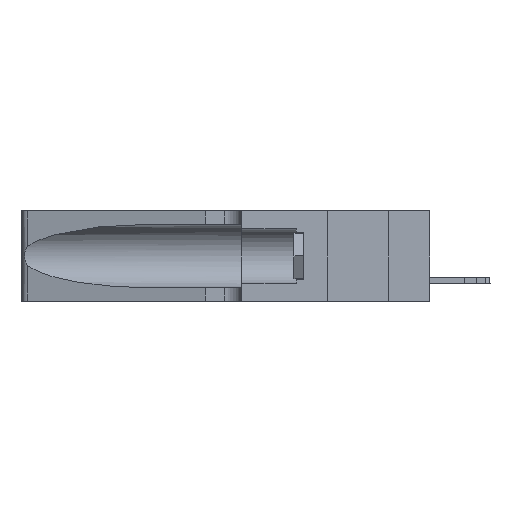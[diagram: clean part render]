
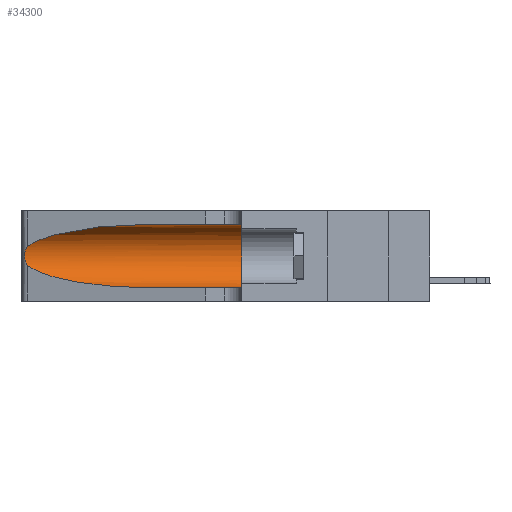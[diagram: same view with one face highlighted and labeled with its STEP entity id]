
A CAD part, left-side view. The second image highlights one B-rep face of the part: STEP entity #34300.
In plain terms, the highlighted cylindrical face has radius 3.308 mm (diameter 6.617 mm), a partial arc.
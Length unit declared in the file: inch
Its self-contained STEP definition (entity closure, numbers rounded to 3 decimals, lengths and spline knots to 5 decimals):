
#672 =( BOUNDED_CURVE ( )  B_SPLINE_CURVE ( 3, ( #29428, #14460, #37527, #17383 ),
 .UNSPECIFIED., .F., .F. ) 
 B_SPLINE_CURVE_WITH_KNOTS ( ( 4, 4 ),
 ( 1.5708, 2.84003 ),
 .UNSPECIFIED. ) 
 CURVE ( )  GEOMETRIC_REPRESENTATION_ITEM ( )  RATIONAL_B_SPLINE_CURVE ( ( 1., 0.87, 0.87, 1. ) ) 
 REPRESENTATION_ITEM ( '' )  );
#2337 = CARTESIAN_POINT ( 'NONE',  ( 0.1305, 1.61858, 0.31525 ) ) ;
#2649 = VERTEX_POINT ( 'NONE', #10686 ) ;
#4021 = CARTESIAN_POINT ( 'NONE',  ( 0.1305, 0.72297, 0.05475 ) ) ;
#5662 = VERTEX_POINT ( 'NONE', #19962 ) ;
#5851 = B_SPLINE_CURVE_WITH_KNOTS ( 'NONE', 3,
 ( #28450, #34926, #15930, #18313, #19242, #28976, #17989, #9977, #15608, #33112, #9560, #18122, #21887, #27722 ),
 .UNSPECIFIED., .F., .F.,
 ( 4, 2, 2, 2, 2, 2, 4 ),
 ( 0., 0.00027, 0.00053, 0.00107, 0.0016, 0.00187, 0.00214 ),
 .UNSPECIFIED. ) ;
#6387 = CARTESIAN_POINT ( 'NONE',  ( 0.1305, 1.61858, 0.185 ) ) ;
#6598 = CIRCLE ( 'NONE', #23271, 0.13025 ) ;
#6604 = ORIENTED_EDGE ( 'NONE', *, *, #36650, .T. ) ;
#7094 = VERTEX_POINT ( 'NONE', #14188 ) ;
#9121 = AXIS2_PLACEMENT_3D ( 'NONE', #6387, #23999, #16027 ) ;
#9560 = CARTESIAN_POINT ( 'NONE',  ( 0.25789, 1.23486, 0.15765 ) ) ;
#9602 = DIRECTION ( 'NONE',  ( 0., 1., 0. ) ) ;
#9977 = CARTESIAN_POINT ( 'NONE',  ( 0.26075, 1.23896, 0.178 ) ) ;
#10686 = CARTESIAN_POINT ( 'NONE',  ( 0.1305, 0.35, 0.05475 ) ) ;
#10847 = EDGE_CURVE ( 'NONE', #5662, #19562, #32777, .T. ) ;
#10902 = DIRECTION ( 'NONE',  ( 0., -1., 0. ) ) ;
#11139 = CARTESIAN_POINT ( 'NONE',  ( 0.1305, 1.61858, 0.05475 ) ) ;
#12680 = CARTESIAN_POINT ( 'NONE',  ( 0.25487, 1.22718, 0.22369 ) ) ;
#14188 = CARTESIAN_POINT ( 'NONE',  ( 0.1305, 0.72297, 0.31525 ) ) ;
#14238 = ORIENTED_EDGE ( 'NONE', *, *, #22538, .T. ) ;
#14460 = CARTESIAN_POINT ( 'NONE',  ( 0.18966, 0.96281, 0.31525 ) ) ;
#14892 = ORIENTED_EDGE ( 'NONE', *, *, #37406, .F. ) ;
#15608 = CARTESIAN_POINT ( 'NONE',  ( 0.26017, 1.23833, 0.17102 ) ) ;
#15930 = CARTESIAN_POINT ( 'NONE',  ( 0.25639, 1.23184, 0.21858 ) ) ;
#16027 = DIRECTION ( 'NONE',  ( 0., 0., -1. ) ) ;
#16653 = DIRECTION ( 'NONE',  ( 0., -1., 0. ) ) ;
#16843 = EDGE_LOOP ( 'NONE', ( #6604, #28564, #25833, #14238, #14892, #31782 ) ) ;
#17383 = CARTESIAN_POINT ( 'NONE',  ( 0.25487, 1.22718, 0.22369 ) ) ;
#17989 = CARTESIAN_POINT ( 'NONE',  ( 0.26075, 1.23896, 0.19203 ) ) ;
#18122 = CARTESIAN_POINT ( 'NONE',  ( 0.25639, 1.23186, 0.15144 ) ) ;
#18313 = CARTESIAN_POINT ( 'NONE',  ( 0.25787, 1.23484, 0.2124 ) ) ;
#18448 = CARTESIAN_POINT ( 'NONE',  ( 0.1305, 0.35, 0.185 ) ) ;
#19175 = CYLINDRICAL_SURFACE ( 'NONE', #9121, 0.13025 ) ;
#19242 = CARTESIAN_POINT ( 'NONE',  ( 0.25854, 1.2359, 0.20912 ) ) ;
#19562 = VERTEX_POINT ( 'NONE', #4021 ) ;
#19962 = CARTESIAN_POINT ( 'NONE',  ( 0.25487, 1.22718, 0.14631 ) ) ;
#20005 = EDGE_CURVE ( 'NONE', #29718, #5662, #5851, .T. ) ;
#20960 = CARTESIAN_POINT ( 'NONE',  ( 0.2373, 1.15595, 0.08982 ) ) ;
#20984 = EDGE_CURVE ( 'NONE', #7094, #26173, #23440, .T. ) ;
#21887 = CARTESIAN_POINT ( 'NONE',  ( 0.25555, 1.22993, 0.14849 ) ) ;
#22048 = VECTOR ( 'NONE', #10902, 39.37008 ) ;
#22538 = EDGE_CURVE ( 'NONE', #19562, #2649, #25653, .T. ) ;
#23271 = AXIS2_PLACEMENT_3D ( 'NONE', #18448, #9602, #24170 ) ;
#23440 = LINE ( 'NONE', #2337, #28058 ) ;
#23727 = CARTESIAN_POINT ( 'NONE',  ( 0.18966, 0.96281, 0.05475 ) ) ;
#23999 = DIRECTION ( 'NONE',  ( 0., -1., 0. ) ) ;
#24170 = DIRECTION ( 'NONE',  ( 0., 0., 1. ) ) ;
#25653 = LINE ( 'NONE', #11139, #22048 ) ;
#25833 = ORIENTED_EDGE ( 'NONE', *, *, #10847, .T. ) ;
#25975 = FACE_OUTER_BOUND ( 'NONE', #16843, .T. ) ;
#26173 = VERTEX_POINT ( 'NONE', #30777 ) ;
#27722 = CARTESIAN_POINT ( 'NONE',  ( 0.25487, 1.22718, 0.14631 ) ) ;
#28058 = VECTOR ( 'NONE', #16653, 39.37008 ) ;
#28450 = CARTESIAN_POINT ( 'NONE',  ( 0.25487, 1.22718, 0.22369 ) ) ;
#28564 = ORIENTED_EDGE ( 'NONE', *, *, #20005, .T. ) ;
#28976 = CARTESIAN_POINT ( 'NONE',  ( 0.26018, 1.23835, 0.19895 ) ) ;
#29428 = CARTESIAN_POINT ( 'NONE',  ( 0.1305, 0.72297, 0.31525 ) ) ;
#29718 = VERTEX_POINT ( 'NONE', #12680 ) ;
#30777 = CARTESIAN_POINT ( 'NONE',  ( 0.1305, 0.35, 0.31525 ) ) ;
#31782 = ORIENTED_EDGE ( 'NONE', *, *, #20984, .F. ) ;
#32463 = CARTESIAN_POINT ( 'NONE',  ( 0.1305, 0.72297, 0.05475 ) ) ;
#32777 =( BOUNDED_CURVE ( )  B_SPLINE_CURVE ( 3, ( #35122, #20960, #23727, #32463 ),
 .UNSPECIFIED., .F., .F. ) 
 B_SPLINE_CURVE_WITH_KNOTS ( ( 4, 4 ),
 ( 3.44316, 4.71239 ),
 .UNSPECIFIED. ) 
 CURVE ( )  GEOMETRIC_REPRESENTATION_ITEM ( )  RATIONAL_B_SPLINE_CURVE ( ( 1., 0.87, 0.87, 1. ) ) 
 REPRESENTATION_ITEM ( '' )  );
#33112 = CARTESIAN_POINT ( 'NONE',  ( 0.25856, 1.23593, 0.16098 ) ) ;
#34300 = ADVANCED_FACE ( 'NONE', ( #25975 ), #19175, .F. ) ;
#34926 = CARTESIAN_POINT ( 'NONE',  ( 0.25555, 1.22994, 0.2215 ) ) ;
#35122 = CARTESIAN_POINT ( 'NONE',  ( 0.25487, 1.22718, 0.14631 ) ) ;
#36650 = EDGE_CURVE ( 'NONE', #7094, #29718, #672, .T. ) ;
#37406 = EDGE_CURVE ( 'NONE', #26173, #2649, #6598, .T. ) ;
#37527 = CARTESIAN_POINT ( 'NONE',  ( 0.2373, 1.15595, 0.28018 ) ) ;
